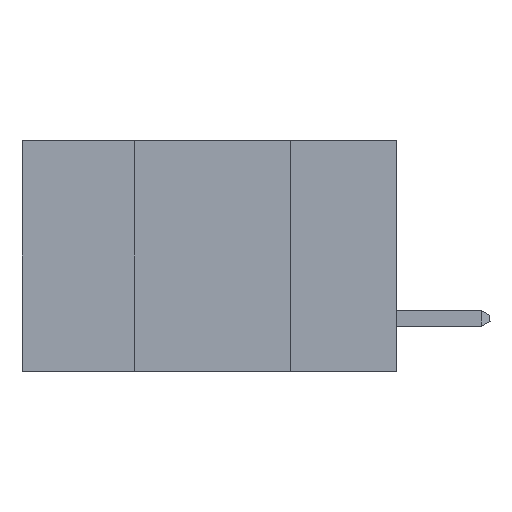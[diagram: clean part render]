
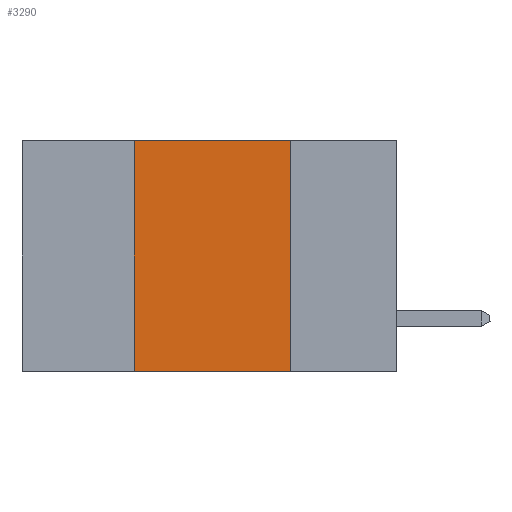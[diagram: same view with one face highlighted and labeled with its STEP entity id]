
A CAD part, left-side view. The second image highlights one B-rep face of the part: STEP entity #3290.
In plain terms, the highlighted planar face has unit normal (-1, 0, 0).
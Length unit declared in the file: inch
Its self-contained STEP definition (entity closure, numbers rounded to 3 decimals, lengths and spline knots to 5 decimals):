
#17 = CARTESIAN_POINT ( 'NONE',  ( 0., 0.42, 0. ) ) ;
#436 = DIRECTION ( 'NONE',  ( 0., -1., 0. ) ) ;
#669 = EDGE_LOOP ( 'NONE', ( #12101, #4264, #1646, #4607 ) ) ;
#1222 = DIRECTION ( 'NONE',  ( 0., 0., 1. ) ) ;
#1310 = VERTEX_POINT ( 'NONE', #8739 ) ;
#1414 = VECTOR ( 'NONE', #11576, 39.37008 ) ;
#1486 = DIRECTION ( 'NONE',  ( 0., -1., 0. ) ) ;
#1576 = LINE ( 'NONE', #6868, #12358 ) ;
#1581 = CARTESIAN_POINT ( 'NONE',  ( 0., 0.6, -0.37 ) ) ;
#1588 = AXIS2_PLACEMENT_3D ( 'NONE', #4477, #5461, #3334 ) ;
#1646 = ORIENTED_EDGE ( 'NONE', *, *, #12363, .F. ) ;
#2391 = LINE ( 'NONE', #1581, #2726 ) ;
#2726 = VECTOR ( 'NONE', #436, 39.37008 ) ;
#2977 = CARTESIAN_POINT ( 'NONE',  ( 0., 0.17, 0. ) ) ;
#3290 = ADVANCED_FACE ( 'NONE', ( #9037 ), #4574, .F. ) ;
#3334 = DIRECTION ( 'NONE',  ( 0., 0., -1. ) ) ;
#3585 = CARTESIAN_POINT ( 'NONE',  ( 0., 0.17, -0.37 ) ) ;
#4027 = LINE ( 'NONE', #4418, #1414 ) ;
#4264 = ORIENTED_EDGE ( 'NONE', *, *, #13355, .F. ) ;
#4418 = CARTESIAN_POINT ( 'NONE',  ( 0., 0.17, 0. ) ) ;
#4477 = CARTESIAN_POINT ( 'NONE',  ( 0., 0.6, 0. ) ) ;
#4574 = PLANE ( 'NONE',  #1588 ) ;
#4607 = ORIENTED_EDGE ( 'NONE', *, *, #11012, .T. ) ;
#4725 = VERTEX_POINT ( 'NONE', #7672 ) ;
#5461 = DIRECTION ( 'NONE',  ( 1., 0., 0. ) ) ;
#6868 = CARTESIAN_POINT ( 'NONE',  ( 0., 0.6, 0. ) ) ;
#7353 = VERTEX_POINT ( 'NONE', #3585 ) ;
#7672 = CARTESIAN_POINT ( 'NONE',  ( 0., 0.42, -0.37 ) ) ;
#7804 = VECTOR ( 'NONE', #1222, 39.37008 ) ;
#8739 = CARTESIAN_POINT ( 'NONE',  ( 0., 0.42, 0. ) ) ;
#9037 = FACE_OUTER_BOUND ( 'NONE', #669, .T. ) ;
#9964 = VERTEX_POINT ( 'NONE', #2977 ) ;
#11012 = EDGE_CURVE ( 'NONE', #4725, #7353, #2391, .T. ) ;
#11576 = DIRECTION ( 'NONE',  ( 0., 0., -1. ) ) ;
#12101 = ORIENTED_EDGE ( 'NONE', *, *, #13014, .F. ) ;
#12358 = VECTOR ( 'NONE', #1486, 39.37008 ) ;
#12363 = EDGE_CURVE ( 'NONE', #4725, #1310, #13143, .T. ) ;
#13014 = EDGE_CURVE ( 'NONE', #9964, #7353, #4027, .T. ) ;
#13143 = LINE ( 'NONE', #17, #7804 ) ;
#13355 = EDGE_CURVE ( 'NONE', #1310, #9964, #1576, .T. ) ;
